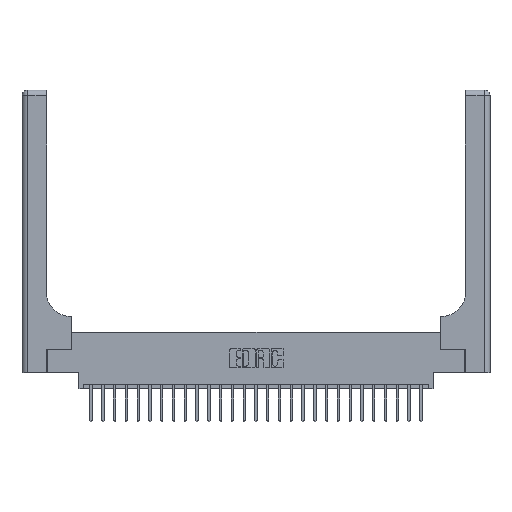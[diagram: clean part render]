
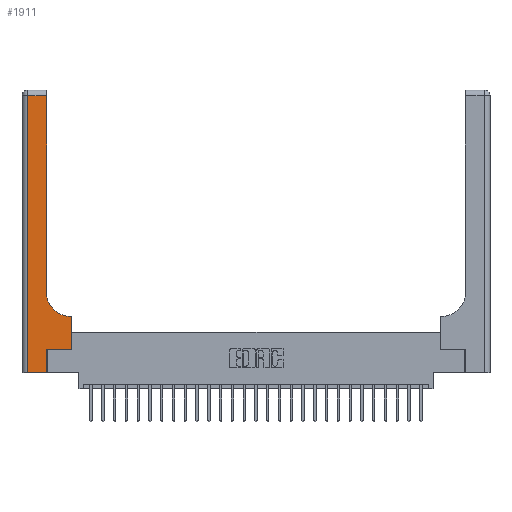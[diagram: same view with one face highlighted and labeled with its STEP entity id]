
A CAD part, top view. The second image highlights one B-rep face of the part: STEP entity #1911.
In plain terms, the highlighted planar face has unit normal (0, 0, 1).
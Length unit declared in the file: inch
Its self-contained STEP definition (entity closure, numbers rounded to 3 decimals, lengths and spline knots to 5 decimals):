
#83 = CARTESIAN_POINT ( 'NONE',  ( 0.06, 0., 0.37 ) ) ;
#642 = DIRECTION ( 'NONE',  ( 0., -1., 0. ) ) ;
#1228 = LINE ( 'NONE', #8996, #11622 ) ;
#1437 = CARTESIAN_POINT ( 'NONE',  ( 0., 2.94, 0.37 ) ) ;
#1911 = ADVANCED_FACE ( 'NONE', ( #22291 ), #8375, .F. ) ;
#2162 = LINE ( 'NONE', #18117, #2345 ) ;
#2345 = VECTOR ( 'NONE', #6183, 39.37008 ) ;
#2417 = CIRCLE ( 'NONE', #22512, 0.25 ) ;
#2536 = LINE ( 'NONE', #23021, #10273 ) ;
#2972 = LINE ( 'NONE', #7123, #9717 ) ;
#3046 = LINE ( 'NONE', #23260, #12711 ) ;
#3162 = CARTESIAN_POINT ( 'NONE',  ( 0.528, 0.6, 0.37 ) ) ;
#3556 = EDGE_CURVE ( 'NONE', #4613, #14497, #2162, .T. ) ;
#3771 = ORIENTED_EDGE ( 'NONE', *, *, #9298, .T. ) ;
#4613 = VERTEX_POINT ( 'NONE', #3162 ) ;
#4793 = CARTESIAN_POINT ( 'NONE',  ( 0.26, 0.85, 0.37 ) ) ;
#5903 = ORIENTED_EDGE ( 'NONE', *, *, #19182, .T. ) ;
#6042 = ORIENTED_EDGE ( 'NONE', *, *, #15535, .T. ) ;
#6183 = DIRECTION ( 'NONE',  ( -1., 0., 0. ) ) ;
#6252 = CARTESIAN_POINT ( 'NONE',  ( 0.06, 2.94, 0.37 ) ) ;
#6857 = DIRECTION ( 'NONE',  ( 0., 1., 0. ) ) ;
#7105 = CARTESIAN_POINT ( 'NONE',  ( 0.26, 2.94, 0.37 ) ) ;
#7123 = CARTESIAN_POINT ( 'NONE',  ( 0.26, 3., 0.37 ) ) ;
#7213 = LINE ( 'NONE', #1437, #11351 ) ;
#7462 = ORIENTED_EDGE ( 'NONE', *, *, #25417, .T. ) ;
#8375 = PLANE ( 'NONE',  #12191 ) ;
#8996 = CARTESIAN_POINT ( 'NONE',  ( 0.528, 0.25, 0.37 ) ) ;
#9036 = CARTESIAN_POINT ( 'NONE',  ( 0.528, 0.25, 0.37 ) ) ;
#9298 = EDGE_CURVE ( 'NONE', #13987, #15811, #2536, .T. ) ;
#9669 = ORIENTED_EDGE ( 'NONE', *, *, #10780, .T. ) ;
#9717 = VECTOR ( 'NONE', #6857, 39.37008 ) ;
#9982 = VECTOR ( 'NONE', #24855, 39.37008 ) ;
#10260 = CARTESIAN_POINT ( 'NONE',  ( 0.265, 0.25, 0.37 ) ) ;
#10273 = VECTOR ( 'NONE', #14847, 39.37008 ) ;
#10780 = EDGE_CURVE ( 'NONE', #19034, #4613, #1228, .T. ) ;
#11351 = VECTOR ( 'NONE', #17129, 39.37008 ) ;
#11622 = VECTOR ( 'NONE', #21303, 39.37008 ) ;
#11841 = DIRECTION ( 'NONE',  ( 1., 0., 0. ) ) ;
#12191 = AXIS2_PLACEMENT_3D ( 'NONE', #12658, #12256, #20423 ) ;
#12256 = DIRECTION ( 'NONE',  ( 0., 0., -1. ) ) ;
#12658 = CARTESIAN_POINT ( 'NONE',  ( 0., 3., 0.37 ) ) ;
#12711 = VECTOR ( 'NONE', #642, 39.37008 ) ;
#12805 = CARTESIAN_POINT ( 'NONE',  ( 0., 0., 0.37 ) ) ;
#12833 = EDGE_LOOP ( 'NONE', ( #17991, #24823, #6042, #22578, #3771, #7462, #9669, #16793, #5903 ) ) ;
#13440 = EDGE_CURVE ( 'NONE', #20126, #13987, #20432, .T. ) ;
#13876 = CARTESIAN_POINT ( 'NONE',  ( 0.265, 0.25, 0.37 ) ) ;
#13987 = VERTEX_POINT ( 'NONE', #21025 ) ;
#14474 = EDGE_CURVE ( 'NONE', #16845, #14752, #7213, .T. ) ;
#14497 = VERTEX_POINT ( 'NONE', #23801 ) ;
#14752 = VERTEX_POINT ( 'NONE', #6252 ) ;
#14847 = DIRECTION ( 'NONE',  ( 0., 1., 0. ) ) ;
#15474 = VERTEX_POINT ( 'NONE', #4793 ) ;
#15535 = EDGE_CURVE ( 'NONE', #14752, #20126, #3046, .T. ) ;
#15811 = VERTEX_POINT ( 'NONE', #13876 ) ;
#15855 = CARTESIAN_POINT ( 'NONE',  ( 0.51, 0.85, 0.37 ) ) ;
#16284 = LINE ( 'NONE', #10260, #16692 ) ;
#16692 = VECTOR ( 'NONE', #20040, 39.37008 ) ;
#16793 = ORIENTED_EDGE ( 'NONE', *, *, #3556, .T. ) ;
#16845 = VERTEX_POINT ( 'NONE', #7105 ) ;
#17129 = DIRECTION ( 'NONE',  ( -1., 0., 0. ) ) ;
#17991 = ORIENTED_EDGE ( 'NONE', *, *, #22339, .T. ) ;
#18117 = CARTESIAN_POINT ( 'NONE',  ( 0.26, 0.6, 0.37 ) ) ;
#19034 = VERTEX_POINT ( 'NONE', #9036 ) ;
#19182 = EDGE_CURVE ( 'NONE', #14497, #15474, #2417, .T. ) ;
#20040 = DIRECTION ( 'NONE',  ( 1., 0., 0. ) ) ;
#20126 = VERTEX_POINT ( 'NONE', #83 ) ;
#20423 = DIRECTION ( 'NONE',  ( -1., 0., 0. ) ) ;
#20432 = LINE ( 'NONE', #12805, #9982 ) ;
#21025 = CARTESIAN_POINT ( 'NONE',  ( 0.265, 0., 0.37 ) ) ;
#21303 = DIRECTION ( 'NONE',  ( 0., 1., 0. ) ) ;
#22291 = FACE_OUTER_BOUND ( 'NONE', #12833, .T. ) ;
#22339 = EDGE_CURVE ( 'NONE', #15474, #16845, #2972, .T. ) ;
#22512 = AXIS2_PLACEMENT_3D ( 'NONE', #15855, #24025, #11841 ) ;
#22578 = ORIENTED_EDGE ( 'NONE', *, *, #13440, .T. ) ;
#23021 = CARTESIAN_POINT ( 'NONE',  ( 0.265, 0., 0.37 ) ) ;
#23260 = CARTESIAN_POINT ( 'NONE',  ( 0.06, 3., 0.37 ) ) ;
#23801 = CARTESIAN_POINT ( 'NONE',  ( 0.51, 0.6, 0.37 ) ) ;
#24025 = DIRECTION ( 'NONE',  ( 0., 0., -1. ) ) ;
#24823 = ORIENTED_EDGE ( 'NONE', *, *, #14474, .T. ) ;
#24855 = DIRECTION ( 'NONE',  ( 1., 0., 0. ) ) ;
#25417 = EDGE_CURVE ( 'NONE', #15811, #19034, #16284, .T. ) ;
